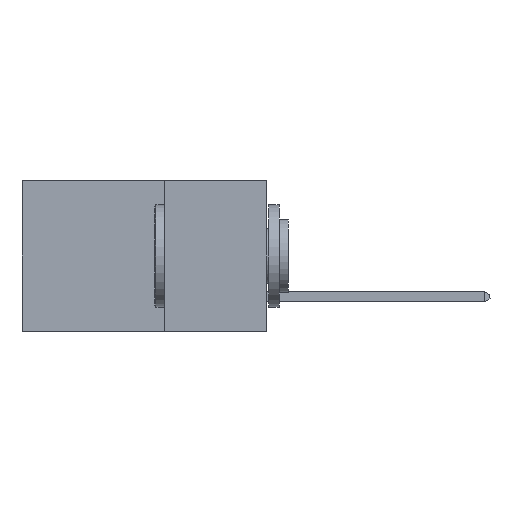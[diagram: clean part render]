
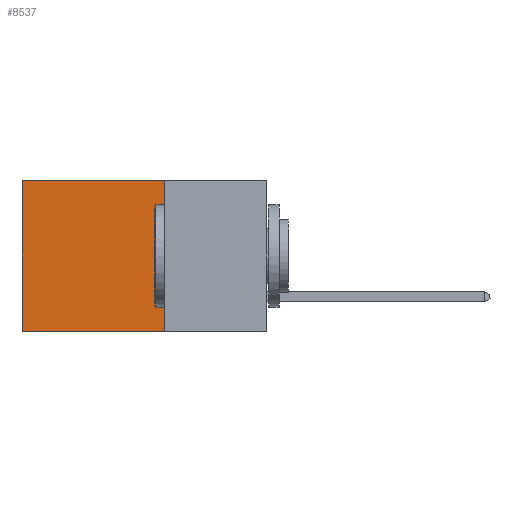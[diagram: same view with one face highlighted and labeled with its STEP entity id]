
A CAD part, left-side view. The second image highlights one B-rep face of the part: STEP entity #8537.
In plain terms, the highlighted planar face has unit normal (-1, 0, 0).
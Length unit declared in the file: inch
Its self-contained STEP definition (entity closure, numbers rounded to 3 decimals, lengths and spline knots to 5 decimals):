
#898 = VERTEX_POINT ( 'NONE', #8362 ) ;
#935 = EDGE_CURVE ( 'NONE', #12267, #898, #11217, .T. ) ;
#1173 = VECTOR ( 'NONE', #1412, 39.37008 ) ;
#1332 = ORIENTED_EDGE ( 'NONE', *, *, #8665, .T. ) ;
#1412 = DIRECTION ( 'NONE',  ( 0., 0., -1. ) ) ;
#1514 = VERTEX_POINT ( 'NONE', #5651 ) ;
#1529 = LINE ( 'NONE', #4607, #1173 ) ;
#2208 = DIRECTION ( 'NONE',  ( 1., 0., 0. ) ) ;
#2432 = DIRECTION ( 'NONE',  ( 0., 0., -1. ) ) ;
#2745 = DIRECTION ( 'NONE',  ( 0., 1., 0. ) ) ;
#2895 = EDGE_CURVE ( 'NONE', #9813, #1514, #5236, .T. ) ;
#2951 = CARTESIAN_POINT ( 'NONE',  ( 0.2875, 0.25, 0. ) ) ;
#3070 = ORIENTED_EDGE ( 'NONE', *, *, #935, .F. ) ;
#4248 = ORIENTED_EDGE ( 'NONE', *, *, #12313, .F. ) ;
#4607 = CARTESIAN_POINT ( 'NONE',  ( 0.2875, 0.25, 0. ) ) ;
#4998 = FACE_OUTER_BOUND ( 'NONE', #8826, .T. ) ;
#5041 = CARTESIAN_POINT ( 'NONE',  ( 0.2875, 0.25, 0. ) ) ;
#5236 = LINE ( 'NONE', #2951, #12747 ) ;
#5453 = DIRECTION ( 'NONE',  ( 0., 1., 0. ) ) ;
#5651 = CARTESIAN_POINT ( 'NONE',  ( 0.2875, 0.6, 0. ) ) ;
#6288 = PLANE ( 'NONE',  #7754 ) ;
#7237 = CARTESIAN_POINT ( 'NONE',  ( 0.2875, 0.25, -0.37 ) ) ;
#7561 = CARTESIAN_POINT ( 'NONE',  ( 0.2875, 0.25, -0.37 ) ) ;
#7676 = ORIENTED_EDGE ( 'NONE', *, *, #2895, .T. ) ;
#7754 = AXIS2_PLACEMENT_3D ( 'NONE', #8343, #2208, #9337 ) ;
#8288 = VECTOR ( 'NONE', #5453, 39.37008 ) ;
#8343 = CARTESIAN_POINT ( 'NONE',  ( 0.2875, 0.25, 0. ) ) ;
#8362 = CARTESIAN_POINT ( 'NONE',  ( 0.2875, 0.6, -0.37 ) ) ;
#8464 = VECTOR ( 'NONE', #2432, 39.37008 ) ;
#8537 = ADVANCED_FACE ( 'NONE', ( #4998 ), #6288, .F. ) ;
#8665 = EDGE_CURVE ( 'NONE', #1514, #898, #11385, .T. ) ;
#8826 = EDGE_LOOP ( 'NONE', ( #1332, #3070, #4248, #7676 ) ) ;
#9337 = DIRECTION ( 'NONE',  ( 0., 0., -1. ) ) ;
#9561 = CARTESIAN_POINT ( 'NONE',  ( 0.2875, 0.6, 0. ) ) ;
#9813 = VERTEX_POINT ( 'NONE', #5041 ) ;
#11217 = LINE ( 'NONE', #7237, #8288 ) ;
#11385 = LINE ( 'NONE', #9561, #8464 ) ;
#12267 = VERTEX_POINT ( 'NONE', #7561 ) ;
#12313 = EDGE_CURVE ( 'NONE', #9813, #12267, #1529, .T. ) ;
#12747 = VECTOR ( 'NONE', #2745, 39.37008 ) ;
